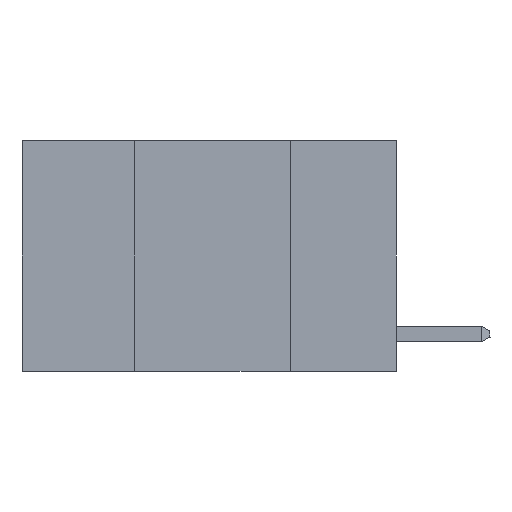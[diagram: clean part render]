
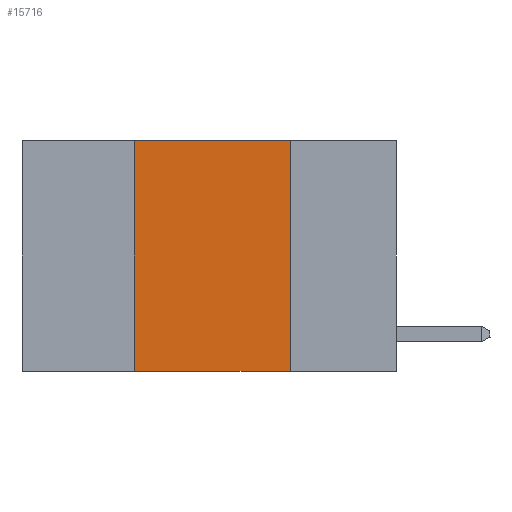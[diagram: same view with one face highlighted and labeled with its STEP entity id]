
A CAD part, left-side view. The second image highlights one B-rep face of the part: STEP entity #15716.
In plain terms, the highlighted planar face has unit normal (-1, 0, 0).
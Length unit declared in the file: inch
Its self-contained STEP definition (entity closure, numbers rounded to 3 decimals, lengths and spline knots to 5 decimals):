
#742 = CARTESIAN_POINT ( 'NONE',  ( 0., 0.17, 0. ) ) ;
#997 = EDGE_CURVE ( 'NONE', #20690, #3854, #3364, .T. ) ;
#2204 = FACE_OUTER_BOUND ( 'NONE', #3597, .T. ) ;
#2275 = DIRECTION ( 'NONE',  ( 0., 0., 1. ) ) ;
#2843 = AXIS2_PLACEMENT_3D ( 'NONE', #13746, #17495, #21352 ) ;
#3364 = LINE ( 'NONE', #22120, #14488 ) ;
#3597 = EDGE_LOOP ( 'NONE', ( #5384, #12862, #17609, #18531 ) ) ;
#3854 = VERTEX_POINT ( 'NONE', #10200 ) ;
#4619 = VECTOR ( 'NONE', #2275, 39.37008 ) ;
#5207 = DIRECTION ( 'NONE',  ( 0., -1., 0. ) ) ;
#5384 = ORIENTED_EDGE ( 'NONE', *, *, #8401, .F. ) ;
#6059 = VERTEX_POINT ( 'NONE', #742 ) ;
#6254 = VECTOR ( 'NONE', #10018, 39.37008 ) ;
#8401 = EDGE_CURVE ( 'NONE', #6059, #3854, #22879, .T. ) ;
#10018 = DIRECTION ( 'NONE',  ( 0., 0., -1. ) ) ;
#10200 = CARTESIAN_POINT ( 'NONE',  ( 0., 0.17, -0.37 ) ) ;
#10979 = LINE ( 'NONE', #18582, #20170 ) ;
#12862 = ORIENTED_EDGE ( 'NONE', *, *, #19488, .F. ) ;
#13531 = CARTESIAN_POINT ( 'NONE',  ( 0., 0.17, 0. ) ) ;
#13746 = CARTESIAN_POINT ( 'NONE',  ( 0., 0.6, 0. ) ) ;
#14488 = VECTOR ( 'NONE', #16496, 39.37008 ) ;
#15115 = CARTESIAN_POINT ( 'NONE',  ( 0., 0.42, 0. ) ) ;
#15550 = CARTESIAN_POINT ( 'NONE',  ( 0., 0.42, 0. ) ) ;
#15716 = ADVANCED_FACE ( 'NONE', ( #2204 ), #15978, .F. ) ;
#15978 = PLANE ( 'NONE',  #2843 ) ;
#16496 = DIRECTION ( 'NONE',  ( 0., -1., 0. ) ) ;
#17046 = LINE ( 'NONE', #15550, #4619 ) ;
#17495 = DIRECTION ( 'NONE',  ( 1., 0., 0. ) ) ;
#17609 = ORIENTED_EDGE ( 'NONE', *, *, #24576, .F. ) ;
#18531 = ORIENTED_EDGE ( 'NONE', *, *, #997, .T. ) ;
#18582 = CARTESIAN_POINT ( 'NONE',  ( 0., 0.6, 0. ) ) ;
#19488 = EDGE_CURVE ( 'NONE', #22616, #6059, #10979, .T. ) ;
#20170 = VECTOR ( 'NONE', #5207, 39.37008 ) ;
#20374 = CARTESIAN_POINT ( 'NONE',  ( 0., 0.42, -0.37 ) ) ;
#20690 = VERTEX_POINT ( 'NONE', #20374 ) ;
#21352 = DIRECTION ( 'NONE',  ( 0., 0., -1. ) ) ;
#22120 = CARTESIAN_POINT ( 'NONE',  ( 0., 0.6, -0.37 ) ) ;
#22616 = VERTEX_POINT ( 'NONE', #15115 ) ;
#22879 = LINE ( 'NONE', #13531, #6254 ) ;
#24576 = EDGE_CURVE ( 'NONE', #20690, #22616, #17046, .T. ) ;
